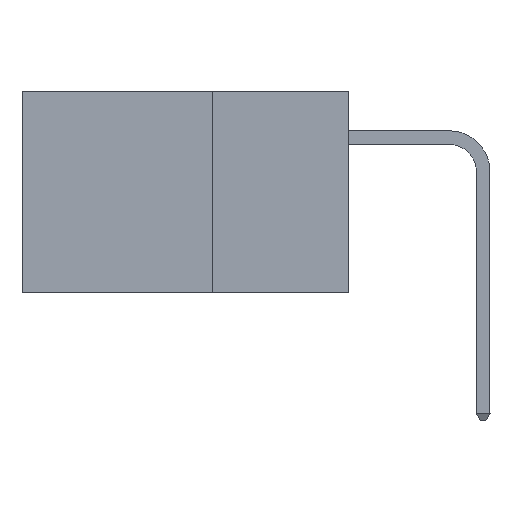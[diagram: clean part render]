
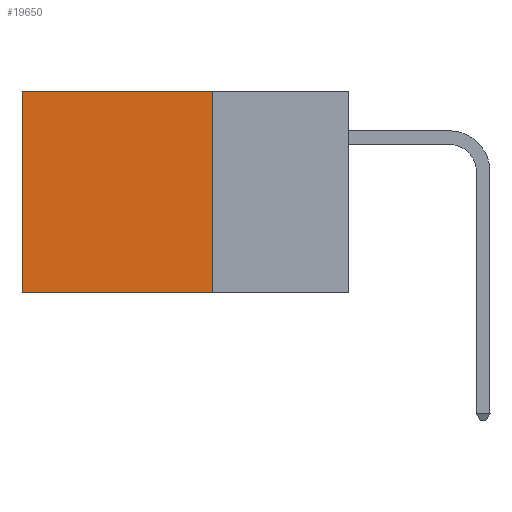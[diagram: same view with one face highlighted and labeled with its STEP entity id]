
A CAD part, left-side view. The second image highlights one B-rep face of the part: STEP entity #19650.
In plain terms, the highlighted planar face has unit normal (-1, 0, 0).
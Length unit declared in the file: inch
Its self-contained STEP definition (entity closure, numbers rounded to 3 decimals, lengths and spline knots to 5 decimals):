
#1263 = CARTESIAN_POINT ( 'NONE',  ( 0.2875, 0.25, -0.37 ) ) ;
#1671 = EDGE_CURVE ( 'NONE', #21925, #3083, #24923, .T. ) ;
#1934 = ORIENTED_EDGE ( 'NONE', *, *, #34743, .F. ) ;
#2076 = DIRECTION ( 'NONE',  ( 0., 0., -1. ) ) ;
#3083 = VERTEX_POINT ( 'NONE', #23176 ) ;
#8923 = EDGE_LOOP ( 'NONE', ( #36349, #34547, #1934, #27798 ) ) ;
#9103 = DIRECTION ( 'NONE',  ( 0., 0., -1. ) ) ;
#11241 = DIRECTION ( 'NONE',  ( 1., 0., 0. ) ) ;
#13621 = CARTESIAN_POINT ( 'NONE',  ( 0.2875, 0.25, 0. ) ) ;
#13674 = LINE ( 'NONE', #16775, #25680 ) ;
#13861 = DIRECTION ( 'NONE',  ( 0., 1., 0. ) ) ;
#14539 = CARTESIAN_POINT ( 'NONE',  ( 0.2875, 0.25, 0. ) ) ;
#14605 = VECTOR ( 'NONE', #17629, 39.37008 ) ;
#16775 = CARTESIAN_POINT ( 'NONE',  ( 0.2875, 0.25, -0.37 ) ) ;
#17629 = DIRECTION ( 'NONE',  ( 0., 0., -1. ) ) ;
#19650 = ADVANCED_FACE ( 'NONE', ( #26176 ), #38193, .F. ) ;
#20589 = CARTESIAN_POINT ( 'NONE',  ( 0.2875, 0.25, 0. ) ) ;
#21331 = VECTOR ( 'NONE', #2076, 39.37008 ) ;
#21925 = VERTEX_POINT ( 'NONE', #26288 ) ;
#23176 = CARTESIAN_POINT ( 'NONE',  ( 0.2875, 0.6, -0.37 ) ) ;
#24923 = LINE ( 'NONE', #25502, #21331 ) ;
#25046 = VERTEX_POINT ( 'NONE', #13621 ) ;
#25502 = CARTESIAN_POINT ( 'NONE',  ( 0.2875, 0.6, 0. ) ) ;
#25680 = VECTOR ( 'NONE', #13861, 39.37008 ) ;
#25981 = LINE ( 'NONE', #34881, #14605 ) ;
#26176 = FACE_OUTER_BOUND ( 'NONE', #8923, .T. ) ;
#26288 = CARTESIAN_POINT ( 'NONE',  ( 0.2875, 0.6, 0. ) ) ;
#27798 = ORIENTED_EDGE ( 'NONE', *, *, #34316, .T. ) ;
#28809 = VECTOR ( 'NONE', #29704, 39.37008 ) ;
#29704 = DIRECTION ( 'NONE',  ( 0., 1., 0. ) ) ;
#32224 = LINE ( 'NONE', #20589, #28809 ) ;
#33703 = AXIS2_PLACEMENT_3D ( 'NONE', #14539, #11241, #9103 ) ;
#33786 = EDGE_CURVE ( 'NONE', #35302, #3083, #13674, .T. ) ;
#34316 = EDGE_CURVE ( 'NONE', #25046, #21925, #32224, .T. ) ;
#34547 = ORIENTED_EDGE ( 'NONE', *, *, #33786, .F. ) ;
#34743 = EDGE_CURVE ( 'NONE', #25046, #35302, #25981, .T. ) ;
#34881 = CARTESIAN_POINT ( 'NONE',  ( 0.2875, 0.25, 0. ) ) ;
#35302 = VERTEX_POINT ( 'NONE', #1263 ) ;
#36349 = ORIENTED_EDGE ( 'NONE', *, *, #1671, .T. ) ;
#38193 = PLANE ( 'NONE',  #33703 ) ;
